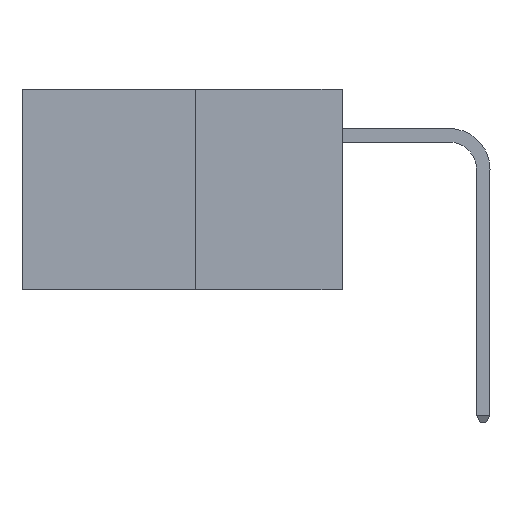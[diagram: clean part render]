
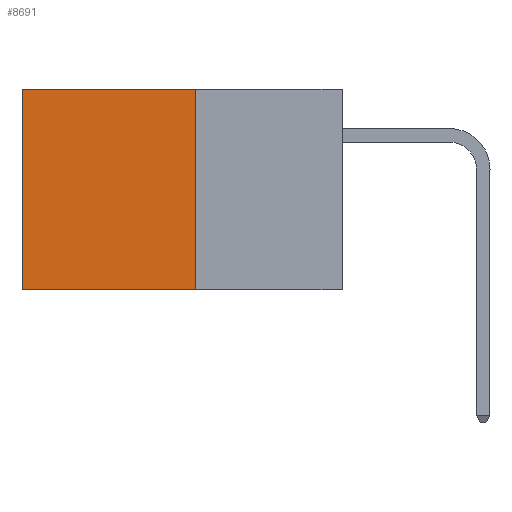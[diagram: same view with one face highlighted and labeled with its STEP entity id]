
A CAD part, left-side view. The second image highlights one B-rep face of the part: STEP entity #8691.
In plain terms, the highlighted planar face has unit normal (-1, 0, 0).
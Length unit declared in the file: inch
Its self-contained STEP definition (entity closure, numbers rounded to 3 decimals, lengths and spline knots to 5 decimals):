
#185 = CARTESIAN_POINT ( 'NONE',  ( 0.277, 0.59, -0.37 ) ) ;
#405 = PLANE ( 'NONE',  #2196 ) ;
#555 = CARTESIAN_POINT ( 'NONE',  ( 0.277, 0.27, 0. ) ) ;
#1118 = CARTESIAN_POINT ( 'NONE',  ( 0.277, 0.27, -0.37 ) ) ;
#1155 = DIRECTION ( 'NONE',  ( 0., 0., -1. ) ) ;
#1402 = CARTESIAN_POINT ( 'NONE',  ( 0.277, 0.27, 0. ) ) ;
#1528 = DIRECTION ( 'NONE',  ( 0., 1., 0. ) ) ;
#2196 = AXIS2_PLACEMENT_3D ( 'NONE', #1118, #5483, #1155 ) ;
#2540 = ORIENTED_EDGE ( 'NONE', *, *, #5101, .F. ) ;
#2764 = EDGE_CURVE ( 'NONE', #2883, #3361, #4691, .T. ) ;
#2883 = VERTEX_POINT ( 'NONE', #555 ) ;
#3137 = VERTEX_POINT ( 'NONE', #8346 ) ;
#3230 = ORIENTED_EDGE ( 'NONE', *, *, #2764, .T. ) ;
#3306 = CARTESIAN_POINT ( 'NONE',  ( 0.277, 0.27, -0.37 ) ) ;
#3361 = VERTEX_POINT ( 'NONE', #7339 ) ;
#3403 = VECTOR ( 'NONE', #1528, 39.37008 ) ;
#3544 = VECTOR ( 'NONE', #6158, 39.37008 ) ;
#3576 = EDGE_LOOP ( 'NONE', ( #6183, #2540, #8528, #3230 ) ) ;
#3646 = CARTESIAN_POINT ( 'NONE',  ( 0.277, 0.59, -0.37 ) ) ;
#3655 = DIRECTION ( 'NONE',  ( 0., 0., -1. ) ) ;
#4091 = EDGE_CURVE ( 'NONE', #3361, #7009, #6865, .T. ) ;
#4691 = LINE ( 'NONE', #1402, #3403 ) ;
#5101 = EDGE_CURVE ( 'NONE', #3137, #7009, #6089, .T. ) ;
#5483 = DIRECTION ( 'NONE',  ( 1., 0., 0. ) ) ;
#5499 = LINE ( 'NONE', #8124, #3544 ) ;
#5877 = VECTOR ( 'NONE', #8786, 39.37008 ) ;
#6089 = LINE ( 'NONE', #3306, #5877 ) ;
#6158 = DIRECTION ( 'NONE',  ( 0., 0., -1. ) ) ;
#6183 = ORIENTED_EDGE ( 'NONE', *, *, #4091, .T. ) ;
#6452 = FACE_OUTER_BOUND ( 'NONE', #3576, .T. ) ;
#6865 = LINE ( 'NONE', #3646, #8564 ) ;
#7009 = VERTEX_POINT ( 'NONE', #185 ) ;
#7339 = CARTESIAN_POINT ( 'NONE',  ( 0.277, 0.59, 0. ) ) ;
#7796 = EDGE_CURVE ( 'NONE', #2883, #3137, #5499, .T. ) ;
#8124 = CARTESIAN_POINT ( 'NONE',  ( 0.277, 0.27, -0.37 ) ) ;
#8346 = CARTESIAN_POINT ( 'NONE',  ( 0.277, 0.27, -0.37 ) ) ;
#8528 = ORIENTED_EDGE ( 'NONE', *, *, #7796, .F. ) ;
#8564 = VECTOR ( 'NONE', #3655, 39.37008 ) ;
#8691 = ADVANCED_FACE ( 'NONE', ( #6452 ), #405, .F. ) ;
#8786 = DIRECTION ( 'NONE',  ( 0., 1., 0. ) ) ;
